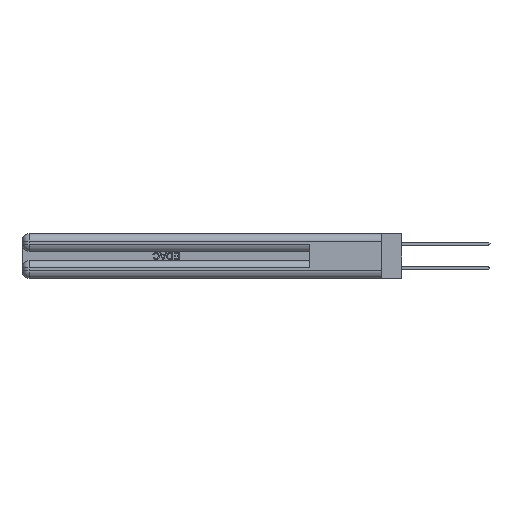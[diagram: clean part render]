
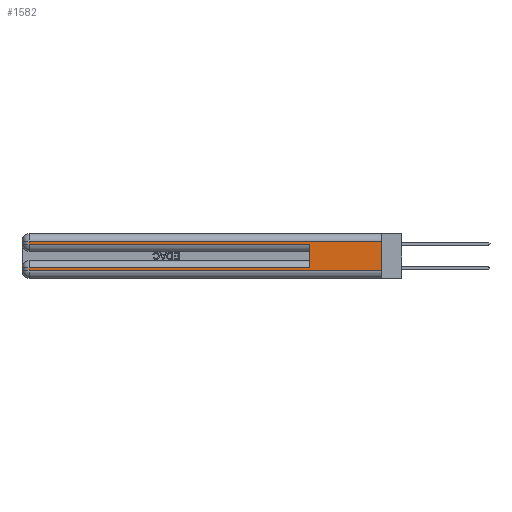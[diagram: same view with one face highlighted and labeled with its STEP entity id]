
A CAD part, left-side view. The second image highlights one B-rep face of the part: STEP entity #1582.
In plain terms, the highlighted planar face has unit normal (-1, 0, 0).
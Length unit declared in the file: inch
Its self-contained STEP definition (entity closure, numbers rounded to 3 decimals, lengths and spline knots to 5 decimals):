
#987 = CARTESIAN_POINT ( 'NONE',  ( 0., 0., 0.37 ) ) ;
#1504 = CARTESIAN_POINT ( 'NONE',  ( 0., 0., 0.06 ) ) ;
#1535 = CARTESIAN_POINT ( 'NONE',  ( 0., 0., 0.37 ) ) ;
#1582 = ADVANCED_FACE ( 'NONE', ( #23595 ), #29921, .F. ) ;
#3657 = VECTOR ( 'NONE', #26157, 39.37008 ) ;
#6561 = CARTESIAN_POINT ( 'NONE',  ( 0., 0., 0.31 ) ) ;
#7484 = VERTEX_POINT ( 'NONE', #52023 ) ;
#8519 = CARTESIAN_POINT ( 'NONE',  ( 0., 0.6, 0.285 ) ) ;
#8661 = DIRECTION ( 'NONE',  ( 0., 0., -1. ) ) ;
#9726 = DIRECTION ( 'NONE',  ( 0., -1., 0. ) ) ;
#11735 = EDGE_CURVE ( 'NONE', #7484, #15528, #19790, .T. ) ;
#12671 = EDGE_CURVE ( 'NONE', #30541, #15528, #33878, .T. ) ;
#12741 = AXIS2_PLACEMENT_3D ( 'NONE', #1535, #33902, #34638 ) ;
#15469 = CARTESIAN_POINT ( 'NONE',  ( 0., 2.94, 0.37 ) ) ;
#15485 = ORIENTED_EDGE ( 'NONE', *, *, #24497, .T. ) ;
#15528 = VERTEX_POINT ( 'NONE', #34905 ) ;
#17175 = CARTESIAN_POINT ( 'NONE',  ( 0., 2.94, 0.31 ) ) ;
#17310 = VERTEX_POINT ( 'NONE', #28948 ) ;
#18171 = CARTESIAN_POINT ( 'NONE',  ( 0., 2.94, 0.06 ) ) ;
#18586 = LINE ( 'NONE', #26973, #21739 ) ;
#19662 = VECTOR ( 'NONE', #50930, 39.37008 ) ;
#19790 = LINE ( 'NONE', #987, #40329 ) ;
#21739 = VECTOR ( 'NONE', #31100, 39.37008 ) ;
#21885 = ORIENTED_EDGE ( 'NONE', *, *, #21941, .T. ) ;
#21941 = EDGE_CURVE ( 'NONE', #24363, #22457, #18586, .T. ) ;
#22222 = CARTESIAN_POINT ( 'NONE',  ( 0., 0.6, 0.145 ) ) ;
#22457 = VERTEX_POINT ( 'NONE', #37946 ) ;
#22944 = VECTOR ( 'NONE', #9726, 39.37008 ) ;
#23595 = FACE_OUTER_BOUND ( 'NONE', #28909, .T. ) ;
#24363 = VERTEX_POINT ( 'NONE', #40055 ) ;
#24497 = EDGE_CURVE ( 'NONE', #22457, #30541, #26631, .T. ) ;
#25638 = ORIENTED_EDGE ( 'NONE', *, *, #31967, .T. ) ;
#26019 = VECTOR ( 'NONE', #31215, 39.37008 ) ;
#26157 = DIRECTION ( 'NONE',  ( 0., 0., 1. ) ) ;
#26631 = LINE ( 'NONE', #15469, #26019 ) ;
#26704 = ORIENTED_EDGE ( 'NONE', *, *, #11735, .F. ) ;
#26973 = CARTESIAN_POINT ( 'NONE',  ( 0., 0., 0.085 ) ) ;
#27410 = EDGE_CURVE ( 'NONE', #17310, #50673, #36392, .T. ) ;
#27503 = ORIENTED_EDGE ( 'NONE', *, *, #12671, .T. ) ;
#28299 = ORIENTED_EDGE ( 'NONE', *, *, #27410, .T. ) ;
#28909 = EDGE_LOOP ( 'NONE', ( #26704, #39050, #25638, #28299, #39581, #21885, #15485, #27503 ) ) ;
#28948 = CARTESIAN_POINT ( 'NONE',  ( 0., 2.94, 0.285 ) ) ;
#29632 = VERTEX_POINT ( 'NONE', #17175 ) ;
#29921 = PLANE ( 'NONE',  #12741 ) ;
#30045 = CARTESIAN_POINT ( 'NONE',  ( 0., 0., 0.285 ) ) ;
#30101 = DIRECTION ( 'NONE',  ( 0., 0., -1. ) ) ;
#30541 = VERTEX_POINT ( 'NONE', #18171 ) ;
#31100 = DIRECTION ( 'NONE',  ( 0., 1., 0. ) ) ;
#31215 = DIRECTION ( 'NONE',  ( 0., 0., -1. ) ) ;
#31747 = LINE ( 'NONE', #6561, #37556 ) ;
#31967 = EDGE_CURVE ( 'NONE', #29632, #17310, #51954, .T. ) ;
#33878 = LINE ( 'NONE', #1504, #22944 ) ;
#33902 = DIRECTION ( 'NONE',  ( 1., 0., 0. ) ) ;
#34638 = DIRECTION ( 'NONE',  ( 0., 0., -1. ) ) ;
#34905 = CARTESIAN_POINT ( 'NONE',  ( 0., 0., 0.06 ) ) ;
#35118 = DIRECTION ( 'NONE',  ( 0., 1., 0. ) ) ;
#36392 = LINE ( 'NONE', #30045, #19662 ) ;
#37103 = EDGE_CURVE ( 'NONE', #7484, #29632, #31747, .T. ) ;
#37556 = VECTOR ( 'NONE', #35118, 39.37008 ) ;
#37946 = CARTESIAN_POINT ( 'NONE',  ( 0., 2.94, 0.085 ) ) ;
#39050 = ORIENTED_EDGE ( 'NONE', *, *, #37103, .T. ) ;
#39581 = ORIENTED_EDGE ( 'NONE', *, *, #43913, .F. ) ;
#40055 = CARTESIAN_POINT ( 'NONE',  ( 0., 0.6, 0.085 ) ) ;
#40329 = VECTOR ( 'NONE', #8661, 39.37008 ) ;
#41045 = VECTOR ( 'NONE', #30101, 39.37008 ) ;
#43913 = EDGE_CURVE ( 'NONE', #24363, #50673, #49174, .T. ) ;
#46517 = CARTESIAN_POINT ( 'NONE',  ( 0., 2.94, 0.37 ) ) ;
#49174 = LINE ( 'NONE', #22222, #3657 ) ;
#50673 = VERTEX_POINT ( 'NONE', #8519 ) ;
#50930 = DIRECTION ( 'NONE',  ( 0., -1., 0. ) ) ;
#51954 = LINE ( 'NONE', #46517, #41045 ) ;
#52023 = CARTESIAN_POINT ( 'NONE',  ( 0., 0., 0.31 ) ) ;
